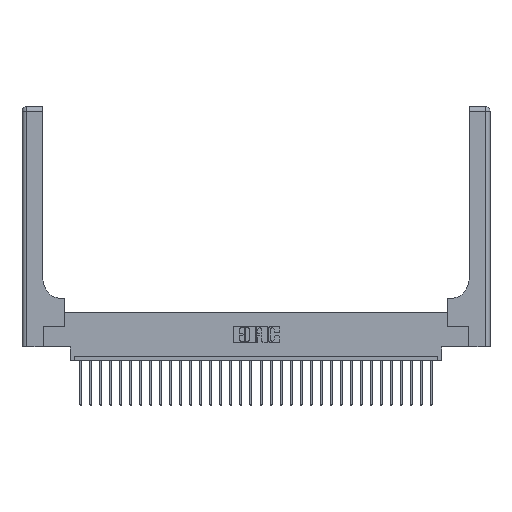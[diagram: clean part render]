
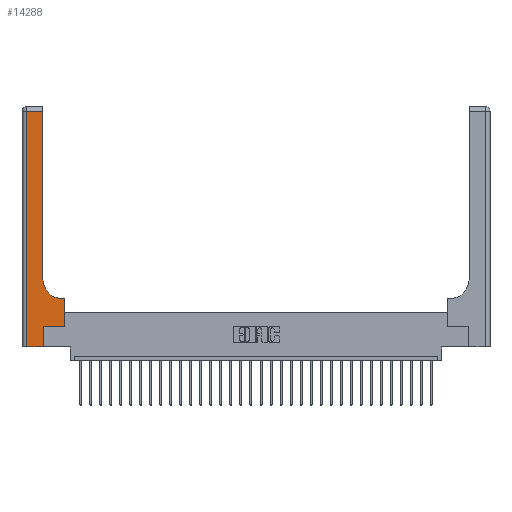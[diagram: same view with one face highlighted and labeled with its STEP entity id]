
A CAD part, top view. The second image highlights one B-rep face of the part: STEP entity #14288.
In plain terms, the highlighted planar face has unit normal (0, 0, 1).
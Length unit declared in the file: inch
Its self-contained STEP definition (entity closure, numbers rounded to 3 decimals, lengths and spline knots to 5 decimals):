
#115 = CARTESIAN_POINT ( 'NONE',  ( 0.06, 3., 0.37 ) ) ;
#270 = VECTOR ( 'NONE', #7170, 39.37008 ) ;
#549 = VERTEX_POINT ( 'NONE', #19344 ) ;
#1532 = CARTESIAN_POINT ( 'NONE',  ( 0.26, 0.6, 0.37 ) ) ;
#1609 = CARTESIAN_POINT ( 'NONE',  ( 0.265, 0., 0.37 ) ) ;
#1622 = DIRECTION ( 'NONE',  ( -1., 0., 0. ) ) ;
#2509 = EDGE_CURVE ( 'NONE', #23047, #11130, #3580, .T. ) ;
#3362 = VERTEX_POINT ( 'NONE', #10439 ) ;
#3580 = LINE ( 'NONE', #19677, #13216 ) ;
#3811 = LINE ( 'NONE', #25006, #20641 ) ;
#4394 = LINE ( 'NONE', #28136, #24011 ) ;
#4748 = VERTEX_POINT ( 'NONE', #21126 ) ;
#5184 = PLANE ( 'NONE',  #21743 ) ;
#5241 = ORIENTED_EDGE ( 'NONE', *, *, #14314, .T. ) ;
#5599 = CARTESIAN_POINT ( 'NONE',  ( 0.26, 0.85, 0.37 ) ) ;
#5798 = CARTESIAN_POINT ( 'NONE',  ( 0.51, 0.85, 0.37 ) ) ;
#6172 = EDGE_CURVE ( 'NONE', #549, #23047, #12357, .T. ) ;
#6270 = CARTESIAN_POINT ( 'NONE',  ( 0.265, 0.25, 0.37 ) ) ;
#6602 = DIRECTION ( 'NONE',  ( 0., -1., 0. ) ) ;
#7170 = DIRECTION ( 'NONE',  ( 1., 0., 0. ) ) ;
#7777 = EDGE_CURVE ( 'NONE', #4748, #3362, #20158, .T. ) ;
#7822 = CARTESIAN_POINT ( 'NONE',  ( 0.528, 0.6, 0.37 ) ) ;
#7830 = LINE ( 'NONE', #1532, #16500 ) ;
#9384 = EDGE_CURVE ( 'NONE', #25416, #4748, #4394, .T. ) ;
#9706 = AXIS2_PLACEMENT_3D ( 'NONE', #5798, #12264, #10017 ) ;
#9968 = DIRECTION ( 'NONE',  ( -1., 0., 0. ) ) ;
#10017 = DIRECTION ( 'NONE',  ( 1., 0., 0. ) ) ;
#10313 = VERTEX_POINT ( 'NONE', #7822 ) ;
#10439 = CARTESIAN_POINT ( 'NONE',  ( 0.528, 0.25, 0.37 ) ) ;
#10558 = VECTOR ( 'NONE', #13202, 39.37008 ) ;
#11130 = VERTEX_POINT ( 'NONE', #15698 ) ;
#11354 = FACE_OUTER_BOUND ( 'NONE', #19195, .T. ) ;
#12264 = DIRECTION ( 'NONE',  ( 0., 0., -1. ) ) ;
#12297 = ORIENTED_EDGE ( 'NONE', *, *, #9384, .T. ) ;
#12357 = CIRCLE ( 'NONE', #9706, 0.25 ) ;
#12583 = ORIENTED_EDGE ( 'NONE', *, *, #6172, .T. ) ;
#12867 = DIRECTION ( 'NONE',  ( 0., 1., 0. ) ) ;
#13202 = DIRECTION ( 'NONE',  ( 1., 0., 0. ) ) ;
#13216 = VECTOR ( 'NONE', #12867, 39.37008 ) ;
#14062 = VECTOR ( 'NONE', #26472, 39.37008 ) ;
#14288 = ADVANCED_FACE ( 'NONE', ( #11354 ), #5184, .F. ) ;
#14314 = EDGE_CURVE ( 'NONE', #11130, #25442, #3811, .T. ) ;
#15275 = EDGE_CURVE ( 'NONE', #10313, #549, #7830, .T. ) ;
#15297 = ORIENTED_EDGE ( 'NONE', *, *, #7777, .T. ) ;
#15698 = CARTESIAN_POINT ( 'NONE',  ( 0.26, 2.94, 0.37 ) ) ;
#16500 = VECTOR ( 'NONE', #1622, 39.37008 ) ;
#16644 = ORIENTED_EDGE ( 'NONE', *, *, #24779, .T. ) ;
#16822 = LINE ( 'NONE', #115, #24702 ) ;
#17491 = VERTEX_POINT ( 'NONE', #18448 ) ;
#18448 = CARTESIAN_POINT ( 'NONE',  ( 0.06, 0., 0.37 ) ) ;
#18664 = DIRECTION ( 'NONE',  ( -1., 0., 0. ) ) ;
#19195 = EDGE_LOOP ( 'NONE', ( #21180, #5241, #21978, #16644, #12297, #15297, #23347, #24895, #12583 ) ) ;
#19344 = CARTESIAN_POINT ( 'NONE',  ( 0.51, 0.6, 0.37 ) ) ;
#19677 = CARTESIAN_POINT ( 'NONE',  ( 0.26, 3., 0.37 ) ) ;
#20004 = EDGE_CURVE ( 'NONE', #3362, #10313, #24713, .T. ) ;
#20158 = LINE ( 'NONE', #6270, #270 ) ;
#20193 = CARTESIAN_POINT ( 'NONE',  ( 0., 3., 0.37 ) ) ;
#20218 = CARTESIAN_POINT ( 'NONE',  ( 0.528, 0.25, 0.37 ) ) ;
#20641 = VECTOR ( 'NONE', #9968, 39.37008 ) ;
#21126 = CARTESIAN_POINT ( 'NONE',  ( 0.265, 0.25, 0.37 ) ) ;
#21180 = ORIENTED_EDGE ( 'NONE', *, *, #2509, .T. ) ;
#21743 = AXIS2_PLACEMENT_3D ( 'NONE', #20193, #22414, #18664 ) ;
#21952 = CARTESIAN_POINT ( 'NONE',  ( 0., 0., 0.37 ) ) ;
#21978 = ORIENTED_EDGE ( 'NONE', *, *, #25084, .T. ) ;
#22414 = DIRECTION ( 'NONE',  ( 0., 0., -1. ) ) ;
#23047 = VERTEX_POINT ( 'NONE', #5599 ) ;
#23219 = CARTESIAN_POINT ( 'NONE',  ( 0.06, 2.94, 0.37 ) ) ;
#23347 = ORIENTED_EDGE ( 'NONE', *, *, #20004, .T. ) ;
#24011 = VECTOR ( 'NONE', #26396, 39.37008 ) ;
#24371 = LINE ( 'NONE', #21952, #10558 ) ;
#24702 = VECTOR ( 'NONE', #6602, 39.37008 ) ;
#24713 = LINE ( 'NONE', #20218, #14062 ) ;
#24779 = EDGE_CURVE ( 'NONE', #17491, #25416, #24371, .T. ) ;
#24895 = ORIENTED_EDGE ( 'NONE', *, *, #15275, .T. ) ;
#25006 = CARTESIAN_POINT ( 'NONE',  ( 0., 2.94, 0.37 ) ) ;
#25084 = EDGE_CURVE ( 'NONE', #25442, #17491, #16822, .T. ) ;
#25416 = VERTEX_POINT ( 'NONE', #1609 ) ;
#25442 = VERTEX_POINT ( 'NONE', #23219 ) ;
#26396 = DIRECTION ( 'NONE',  ( 0., 1., 0. ) ) ;
#26472 = DIRECTION ( 'NONE',  ( 0., 1., 0. ) ) ;
#28136 = CARTESIAN_POINT ( 'NONE',  ( 0.265, 0., 0.37 ) ) ;
